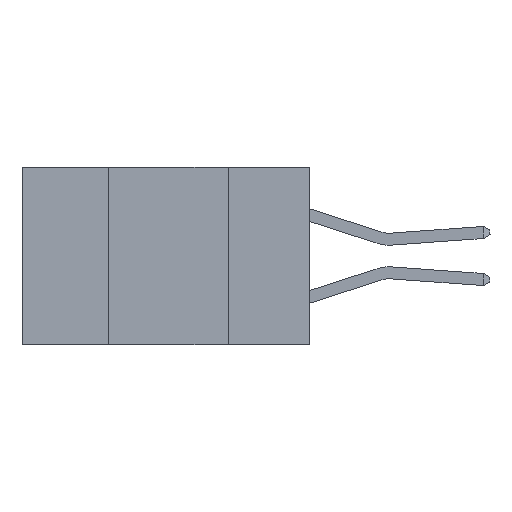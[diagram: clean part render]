
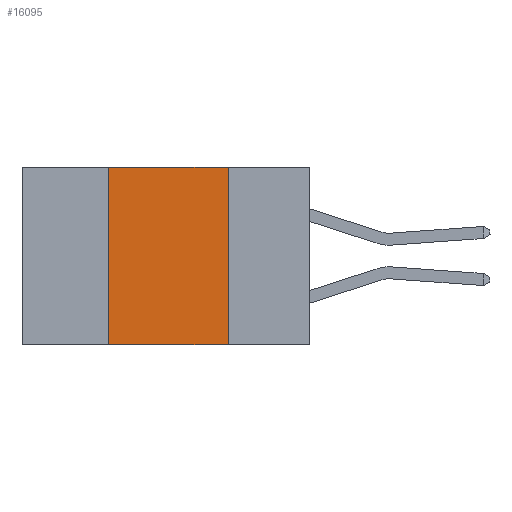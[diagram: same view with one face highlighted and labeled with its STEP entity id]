
A CAD part, left-side view. The second image highlights one B-rep face of the part: STEP entity #16095.
In plain terms, the highlighted planar face has unit normal (-1, 0, 0).
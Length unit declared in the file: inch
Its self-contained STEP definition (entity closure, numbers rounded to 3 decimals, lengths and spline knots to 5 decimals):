
#53 = ORIENTED_EDGE ( 'NONE', *, *, #15439, .F. ) ;
#81 = DIRECTION ( 'NONE',  ( 1., 0., 0. ) ) ;
#586 = CARTESIAN_POINT ( 'NONE',  ( 0., 0.42, 0. ) ) ;
#740 = EDGE_CURVE ( 'NONE', #3432, #7502, #5269, .T. ) ;
#1502 = DIRECTION ( 'NONE',  ( 0., -1., 0. ) ) ;
#1817 = VECTOR ( 'NONE', #3077, 39.37008 ) ;
#2017 = AXIS2_PLACEMENT_3D ( 'NONE', #15319, #81, #9142 ) ;
#2229 = VECTOR ( 'NONE', #1502, 39.37008 ) ;
#3047 = LINE ( 'NONE', #10430, #2229 ) ;
#3077 = DIRECTION ( 'NONE',  ( 0., 0., -1. ) ) ;
#3334 = LINE ( 'NONE', #3335, #16293 ) ;
#3335 = CARTESIAN_POINT ( 'NONE',  ( 0., 0.42, -0.37 ) ) ;
#3432 = VERTEX_POINT ( 'NONE', #14832 ) ;
#4002 = LINE ( 'NONE', #12019, #16160 ) ;
#4634 = DIRECTION ( 'NONE',  ( 0., 0., 1. ) ) ;
#4865 = VERTEX_POINT ( 'NONE', #586 ) ;
#5269 = LINE ( 'NONE', #15065, #1817 ) ;
#5821 = ORIENTED_EDGE ( 'NONE', *, *, #740, .F. ) ;
#6238 = EDGE_CURVE ( 'NONE', #9325, #7502, #4002, .T. ) ;
#6592 = PLANE ( 'NONE',  #2017 ) ;
#6985 = ORIENTED_EDGE ( 'NONE', *, *, #13781, .F. ) ;
#7502 = VERTEX_POINT ( 'NONE', #15443 ) ;
#9116 = EDGE_LOOP ( 'NONE', ( #5821, #53, #6985, #13454 ) ) ;
#9142 = DIRECTION ( 'NONE',  ( 0., 0., -1. ) ) ;
#9325 = VERTEX_POINT ( 'NONE', #9531 ) ;
#9531 = CARTESIAN_POINT ( 'NONE',  ( 0., 0.42, -0.37 ) ) ;
#9561 = FACE_OUTER_BOUND ( 'NONE', #9116, .T. ) ;
#10430 = CARTESIAN_POINT ( 'NONE',  ( 0., 0.6, 0. ) ) ;
#12019 = CARTESIAN_POINT ( 'NONE',  ( 0., 0.6, -0.37 ) ) ;
#13222 = DIRECTION ( 'NONE',  ( 0., -1., 0. ) ) ;
#13454 = ORIENTED_EDGE ( 'NONE', *, *, #6238, .T. ) ;
#13781 = EDGE_CURVE ( 'NONE', #9325, #4865, #3334, .T. ) ;
#14832 = CARTESIAN_POINT ( 'NONE',  ( 0., 0.17, 0. ) ) ;
#15065 = CARTESIAN_POINT ( 'NONE',  ( 0., 0.17, -0.37 ) ) ;
#15319 = CARTESIAN_POINT ( 'NONE',  ( 0., 0.6, 0. ) ) ;
#15439 = EDGE_CURVE ( 'NONE', #4865, #3432, #3047, .T. ) ;
#15443 = CARTESIAN_POINT ( 'NONE',  ( 0., 0.17, -0.37 ) ) ;
#16095 = ADVANCED_FACE ( 'NONE', ( #9561 ), #6592, .F. ) ;
#16160 = VECTOR ( 'NONE', #13222, 39.37008 ) ;
#16293 = VECTOR ( 'NONE', #4634, 39.37008 ) ;
